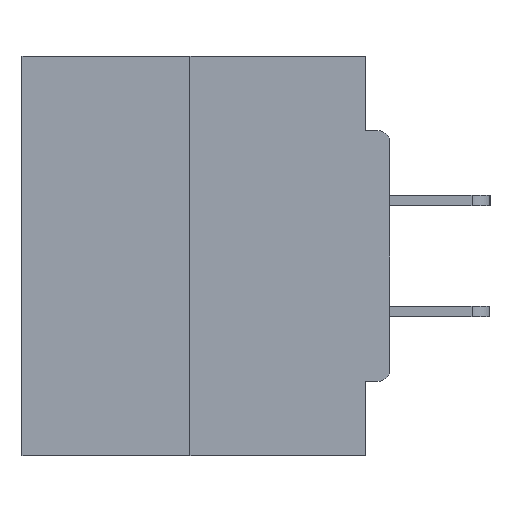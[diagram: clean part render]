
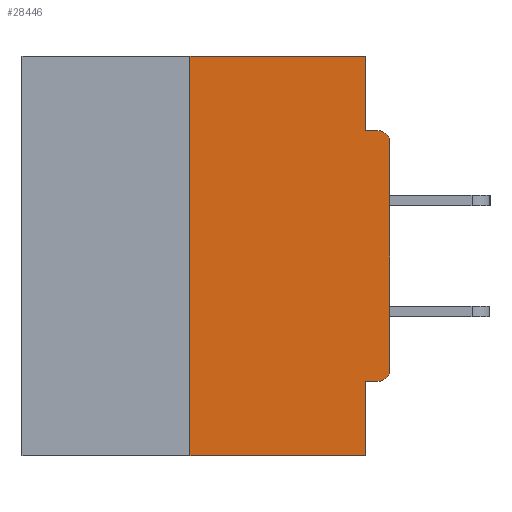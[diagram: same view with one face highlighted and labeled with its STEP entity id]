
A CAD part, left-side view. The second image highlights one B-rep face of the part: STEP entity #28446.
In plain terms, the highlighted planar face has unit normal (-1, 0, 0).
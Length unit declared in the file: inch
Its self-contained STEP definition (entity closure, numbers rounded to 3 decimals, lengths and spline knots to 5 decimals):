
#685 = LINE ( 'NONE', #10581, #27987 ) ;
#1782 = EDGE_LOOP ( 'NONE', ( #20476, #34149, #31076, #28176, #7074, #19615, #33294, #30173, #8601, #11351 ) ) ;
#1908 = FACE_OUTER_BOUND ( 'NONE', #1782, .T. ) ;
#1971 = VECTOR ( 'NONE', #14419, 39.37008 ) ;
#2486 = LINE ( 'NONE', #6518, #31862 ) ;
#3681 = CARTESIAN_POINT ( 'NONE',  ( 0., 0., -0.3915 ) ) ;
#3779 = CARTESIAN_POINT ( 'NONE',  ( 0., 0.25, -0.5 ) ) ;
#4706 = CIRCLE ( 'NONE', #21343, 0.015 ) ;
#5281 = LINE ( 'NONE', #27699, #1971 ) ;
#5892 = EDGE_CURVE ( 'NONE', #12417, #13171, #685, .T. ) ;
#6345 = CARTESIAN_POINT ( 'NONE',  ( 0., 0.031, -0.4065 ) ) ;
#6419 = CARTESIAN_POINT ( 'NONE',  ( 0., 0.015, -0.0935 ) ) ;
#6518 = CARTESIAN_POINT ( 'NONE',  ( 0., 0.46, -0.5 ) ) ;
#6736 = CARTESIAN_POINT ( 'NONE',  ( 0., 0.25, 0. ) ) ;
#6871 = LINE ( 'NONE', #27058, #13895 ) ;
#7074 = ORIENTED_EDGE ( 'NONE', *, *, #28903, .F. ) ;
#7482 = EDGE_CURVE ( 'NONE', #29145, #12001, #34107, .T. ) ;
#7734 = CARTESIAN_POINT ( 'NONE',  ( 0., 0.015, -0.4065 ) ) ;
#7915 = CARTESIAN_POINT ( 'NONE',  ( 0., 0.031, 0. ) ) ;
#8503 = DIRECTION ( 'NONE',  ( 0., -1., 0. ) ) ;
#8601 = ORIENTED_EDGE ( 'NONE', *, *, #21460, .F. ) ;
#9404 = DIRECTION ( 'NONE',  ( -1., 0., 0. ) ) ;
#10540 = VECTOR ( 'NONE', #18352, 39.37008 ) ;
#10581 = CARTESIAN_POINT ( 'NONE',  ( 0., 0., 0. ) ) ;
#11338 = DIRECTION ( 'NONE',  ( 0., 1., 0. ) ) ;
#11351 = ORIENTED_EDGE ( 'NONE', *, *, #30901, .F. ) ;
#11593 = CARTESIAN_POINT ( 'NONE',  ( 0., 0.015, -0.3915 ) ) ;
#11928 = VECTOR ( 'NONE', #33785, 39.37008 ) ;
#12001 = VERTEX_POINT ( 'NONE', #27629 ) ;
#12051 = DIRECTION ( 'NONE',  ( 0., 0., -1. ) ) ;
#12077 = VERTEX_POINT ( 'NONE', #7734 ) ;
#12274 = CARTESIAN_POINT ( 'NONE',  ( 0., 0.015, -0.1085 ) ) ;
#12417 = VERTEX_POINT ( 'NONE', #3681 ) ;
#13171 = VERTEX_POINT ( 'NONE', #15352 ) ;
#13451 = DIRECTION ( 'NONE',  ( 0., 0., 1. ) ) ;
#13895 = VECTOR ( 'NONE', #11338, 39.37008 ) ;
#14419 = DIRECTION ( 'NONE',  ( 0., 0., 1. ) ) ;
#15100 = VERTEX_POINT ( 'NONE', #6419 ) ;
#15352 = CARTESIAN_POINT ( 'NONE',  ( 0., 0., -0.1085 ) ) ;
#16022 = LINE ( 'NONE', #20698, #11928 ) ;
#16984 = AXIS2_PLACEMENT_3D ( 'NONE', #28332, #28106, #30998 ) ;
#17657 = EDGE_CURVE ( 'NONE', #12077, #12417, #27436, .T. ) ;
#17673 = EDGE_CURVE ( 'NONE', #30368, #28083, #23307, .T. ) ;
#18352 = DIRECTION ( 'NONE',  ( 0., 0., -1. ) ) ;
#19615 = ORIENTED_EDGE ( 'NONE', *, *, #17657, .T. ) ;
#19901 = EDGE_CURVE ( 'NONE', #33339, #12001, #2486, .T. ) ;
#20476 = ORIENTED_EDGE ( 'NONE', *, *, #17673, .F. ) ;
#20698 = CARTESIAN_POINT ( 'NONE',  ( 0., 0., -0.0935 ) ) ;
#21158 = CARTESIAN_POINT ( 'NONE',  ( 0., 0.031, 0. ) ) ;
#21270 = DIRECTION ( 'NONE',  ( 0., 0., -1. ) ) ;
#21343 = AXIS2_PLACEMENT_3D ( 'NONE', #12274, #9404, #12051 ) ;
#21349 = EDGE_CURVE ( 'NONE', #33339, #30368, #5281, .T. ) ;
#21460 = EDGE_CURVE ( 'NONE', #31318, #15100, #16022, .T. ) ;
#23135 = AXIS2_PLACEMENT_3D ( 'NONE', #11593, #24343, #32659 ) ;
#23307 = LINE ( 'NONE', #30112, #29941 ) ;
#24343 = DIRECTION ( 'NONE',  ( -1., 0., 0. ) ) ;
#27022 = VECTOR ( 'NONE', #21270, 39.37008 ) ;
#27058 = CARTESIAN_POINT ( 'NONE',  ( 0., 0., -0.4065 ) ) ;
#27436 = CIRCLE ( 'NONE', #23135, 0.015 ) ;
#27629 = CARTESIAN_POINT ( 'NONE',  ( 0., 0.031, -0.5 ) ) ;
#27645 = DIRECTION ( 'NONE',  ( 0., -1., 0. ) ) ;
#27699 = CARTESIAN_POINT ( 'NONE',  ( 0., 0.25, 0. ) ) ;
#27987 = VECTOR ( 'NONE', #13451, 39.37008 ) ;
#28083 = VERTEX_POINT ( 'NONE', #7915 ) ;
#28106 = DIRECTION ( 'NONE',  ( 1., 0., 0. ) ) ;
#28176 = ORIENTED_EDGE ( 'NONE', *, *, #7482, .F. ) ;
#28332 = CARTESIAN_POINT ( 'NONE',  ( 0., 0.46, 0. ) ) ;
#28446 = ADVANCED_FACE ( 'NONE', ( #1908 ), #30666, .F. ) ;
#28903 = EDGE_CURVE ( 'NONE', #12077, #29145, #6871, .T. ) ;
#29129 = CARTESIAN_POINT ( 'NONE',  ( 0., 0.031, -0.5 ) ) ;
#29145 = VERTEX_POINT ( 'NONE', #6345 ) ;
#29941 = VECTOR ( 'NONE', #8503, 39.37008 ) ;
#30112 = CARTESIAN_POINT ( 'NONE',  ( 0., 0.46, 0. ) ) ;
#30173 = ORIENTED_EDGE ( 'NONE', *, *, #30654, .T. ) ;
#30368 = VERTEX_POINT ( 'NONE', #6736 ) ;
#30654 = EDGE_CURVE ( 'NONE', #13171, #15100, #4706, .T. ) ;
#30666 = PLANE ( 'NONE',  #16984 ) ;
#30901 = EDGE_CURVE ( 'NONE', #28083, #31318, #34044, .T. ) ;
#30972 = CARTESIAN_POINT ( 'NONE',  ( 0., 0.031, -0.0935 ) ) ;
#30998 = DIRECTION ( 'NONE',  ( 0., 0., -1. ) ) ;
#31076 = ORIENTED_EDGE ( 'NONE', *, *, #19901, .T. ) ;
#31318 = VERTEX_POINT ( 'NONE', #30972 ) ;
#31862 = VECTOR ( 'NONE', #27645, 39.37008 ) ;
#32659 = DIRECTION ( 'NONE',  ( 0., 0., -1. ) ) ;
#33294 = ORIENTED_EDGE ( 'NONE', *, *, #5892, .T. ) ;
#33339 = VERTEX_POINT ( 'NONE', #3779 ) ;
#33785 = DIRECTION ( 'NONE',  ( 0., -1., 0. ) ) ;
#34044 = LINE ( 'NONE', #21158, #27022 ) ;
#34107 = LINE ( 'NONE', #29129, #10540 ) ;
#34149 = ORIENTED_EDGE ( 'NONE', *, *, #21349, .F. ) ;
